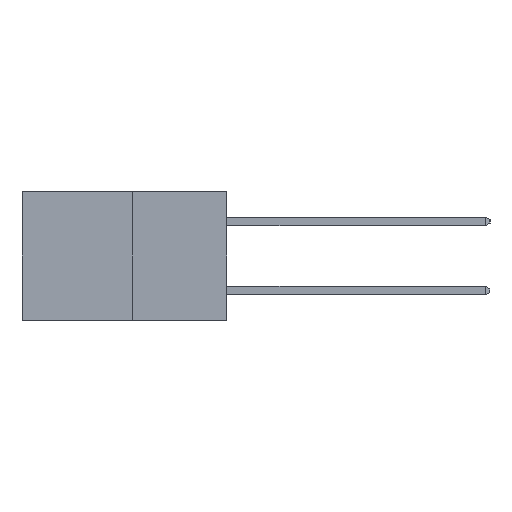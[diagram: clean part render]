
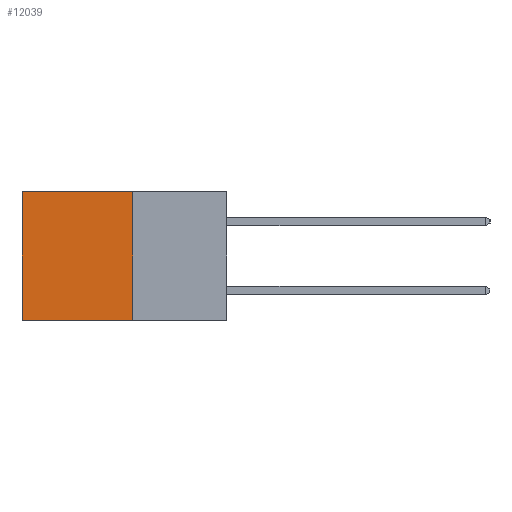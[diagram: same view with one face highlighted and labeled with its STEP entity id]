
A CAD part, left-side view. The second image highlights one B-rep face of the part: STEP entity #12039.
In plain terms, the highlighted planar face has unit normal (-1, 0, 0).
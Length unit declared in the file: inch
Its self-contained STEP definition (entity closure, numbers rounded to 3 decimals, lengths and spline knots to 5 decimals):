
#8 = DIRECTION ( 'NONE',  ( 0., 1., 0. ) ) ;
#206 = DIRECTION ( 'NONE',  ( 0., 0., -1. ) ) ;
#856 = LINE ( 'NONE', #10095, #13772 ) ;
#1221 = CARTESIAN_POINT ( 'NONE',  ( 0.277, 0.27, -0.37 ) ) ;
#1329 = CARTESIAN_POINT ( 'NONE',  ( 0.277, 0.27, -0.37 ) ) ;
#1848 = CARTESIAN_POINT ( 'NONE',  ( 0.277, 0.27, -0.37 ) ) ;
#2561 = DIRECTION ( 'NONE',  ( 1., 0., 0. ) ) ;
#3623 = LINE ( 'NONE', #13033, #10204 ) ;
#3776 = ORIENTED_EDGE ( 'NONE', *, *, #7692, .T. ) ;
#4311 = ORIENTED_EDGE ( 'NONE', *, *, #14071, .F. ) ;
#4417 = VECTOR ( 'NONE', #8, 39.37008 ) ;
#5198 = VERTEX_POINT ( 'NONE', #11449 ) ;
#5793 = FACE_OUTER_BOUND ( 'NONE', #15175, .T. ) ;
#6451 = EDGE_CURVE ( 'NONE', #11824, #8555, #856, .T. ) ;
#6832 = CARTESIAN_POINT ( 'NONE',  ( 0.277, 0.59, -0.37 ) ) ;
#7354 = LINE ( 'NONE', #1848, #10386 ) ;
#7692 = EDGE_CURVE ( 'NONE', #5198, #11824, #3623, .T. ) ;
#7885 = PLANE ( 'NONE',  #10834 ) ;
#7946 = LINE ( 'NONE', #1221, #4417 ) ;
#8555 = VERTEX_POINT ( 'NONE', #6832 ) ;
#9090 = ORIENTED_EDGE ( 'NONE', *, *, #9097, .F. ) ;
#9097 = EDGE_CURVE ( 'NONE', #5198, #15476, #7354, .T. ) ;
#9607 = ORIENTED_EDGE ( 'NONE', *, *, #6451, .T. ) ;
#10095 = CARTESIAN_POINT ( 'NONE',  ( 0.277, 0.59, -0.37 ) ) ;
#10204 = VECTOR ( 'NONE', #12635, 39.37008 ) ;
#10386 = VECTOR ( 'NONE', #14969, 39.37008 ) ;
#10834 = AXIS2_PLACEMENT_3D ( 'NONE', #11667, #2561, #11714 ) ;
#11333 = CARTESIAN_POINT ( 'NONE',  ( 0.277, 0.59, 0. ) ) ;
#11449 = CARTESIAN_POINT ( 'NONE',  ( 0.277, 0.27, 0. ) ) ;
#11667 = CARTESIAN_POINT ( 'NONE',  ( 0.277, 0.27, -0.37 ) ) ;
#11714 = DIRECTION ( 'NONE',  ( 0., 0., -1. ) ) ;
#11824 = VERTEX_POINT ( 'NONE', #11333 ) ;
#12039 = ADVANCED_FACE ( 'NONE', ( #5793 ), #7885, .F. ) ;
#12635 = DIRECTION ( 'NONE',  ( 0., 1., 0. ) ) ;
#13033 = CARTESIAN_POINT ( 'NONE',  ( 0.277, 0.27, 0. ) ) ;
#13772 = VECTOR ( 'NONE', #206, 39.37008 ) ;
#14071 = EDGE_CURVE ( 'NONE', #15476, #8555, #7946, .T. ) ;
#14969 = DIRECTION ( 'NONE',  ( 0., 0., -1. ) ) ;
#15175 = EDGE_LOOP ( 'NONE', ( #9607, #4311, #9090, #3776 ) ) ;
#15476 = VERTEX_POINT ( 'NONE', #1329 ) ;
